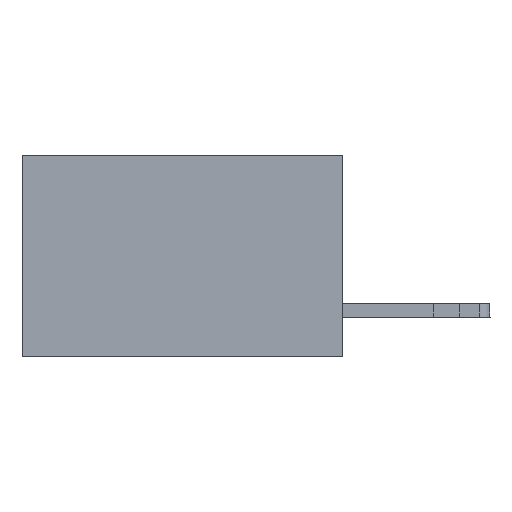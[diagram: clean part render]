
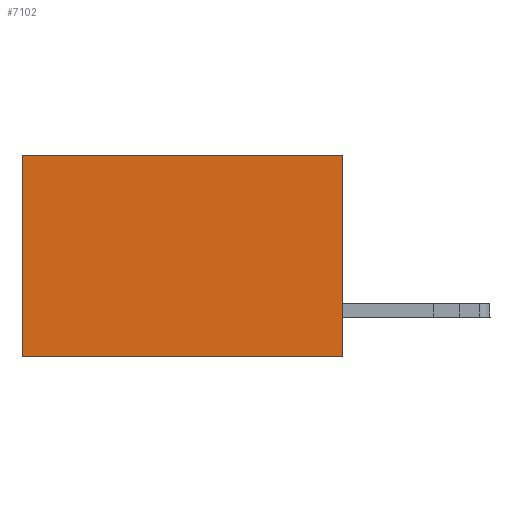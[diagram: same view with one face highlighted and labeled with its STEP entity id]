
A CAD part, left-side view. The second image highlights one B-rep face of the part: STEP entity #7102.
In plain terms, the highlighted planar face has unit normal (-1, 0, 0).
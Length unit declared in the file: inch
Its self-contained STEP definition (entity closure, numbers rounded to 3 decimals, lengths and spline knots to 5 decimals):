
#119 = VECTOR ( 'NONE', #19900, 39.37008 ) ;
#282 = CARTESIAN_POINT ( 'NONE',  ( 0.277, 0.59, -0.37 ) ) ;
#523 = AXIS2_PLACEMENT_3D ( 'NONE', #13815, #13950, #26799 ) ;
#1817 = DIRECTION ( 'NONE',  ( 0., 1., 0. ) ) ;
#3005 = VERTEX_POINT ( 'NONE', #25393 ) ;
#3734 = PLANE ( 'NONE',  #523 ) ;
#4104 = CARTESIAN_POINT ( 'NONE',  ( 0.277, 0., -0.37 ) ) ;
#4737 = LINE ( 'NONE', #19126, #23913 ) ;
#5538 = ORIENTED_EDGE ( 'NONE', *, *, #11584, .T. ) ;
#6023 = CARTESIAN_POINT ( 'NONE',  ( 0.277, 0., 0. ) ) ;
#7102 = ADVANCED_FACE ( 'NONE', ( #22866 ), #3734, .F. ) ;
#7572 = CARTESIAN_POINT ( 'NONE',  ( 0.277, 0.59, -0.37 ) ) ;
#8083 = EDGE_CURVE ( 'NONE', #23584, #9351, #11392, .T. ) ;
#8929 = ORIENTED_EDGE ( 'NONE', *, *, #21831, .T. ) ;
#9351 = VERTEX_POINT ( 'NONE', #4104 ) ;
#10187 = ORIENTED_EDGE ( 'NONE', *, *, #8083, .F. ) ;
#10646 = LINE ( 'NONE', #282, #11764 ) ;
#10917 = DIRECTION ( 'NONE',  ( 0., 0., -1. ) ) ;
#11392 = LINE ( 'NONE', #20463, #119 ) ;
#11495 = EDGE_LOOP ( 'NONE', ( #5538, #24418, #10187, #8929 ) ) ;
#11584 = EDGE_CURVE ( 'NONE', #3005, #13792, #10646, .T. ) ;
#11764 = VECTOR ( 'NONE', #10917, 39.37008 ) ;
#12848 = DIRECTION ( 'NONE',  ( 0., 1., 0. ) ) ;
#13792 = VERTEX_POINT ( 'NONE', #7572 ) ;
#13797 = VECTOR ( 'NONE', #1817, 39.37008 ) ;
#13815 = CARTESIAN_POINT ( 'NONE',  ( 0.277, 0., -0.37 ) ) ;
#13950 = DIRECTION ( 'NONE',  ( 1., 0., 0. ) ) ;
#16779 = LINE ( 'NONE', #6023, #13797 ) ;
#19126 = CARTESIAN_POINT ( 'NONE',  ( 0.277, 0., -0.37 ) ) ;
#19660 = CARTESIAN_POINT ( 'NONE',  ( 0.277, 0., 0. ) ) ;
#19900 = DIRECTION ( 'NONE',  ( 0., 0., -1. ) ) ;
#20463 = CARTESIAN_POINT ( 'NONE',  ( 0.277, 0., -0.37 ) ) ;
#21831 = EDGE_CURVE ( 'NONE', #23584, #3005, #16779, .T. ) ;
#22866 = FACE_OUTER_BOUND ( 'NONE', #11495, .T. ) ;
#23584 = VERTEX_POINT ( 'NONE', #19660 ) ;
#23913 = VECTOR ( 'NONE', #12848, 39.37008 ) ;
#24418 = ORIENTED_EDGE ( 'NONE', *, *, #25938, .F. ) ;
#25393 = CARTESIAN_POINT ( 'NONE',  ( 0.277, 0.59, 0. ) ) ;
#25938 = EDGE_CURVE ( 'NONE', #9351, #13792, #4737, .T. ) ;
#26799 = DIRECTION ( 'NONE',  ( 0., 0., -1. ) ) ;
